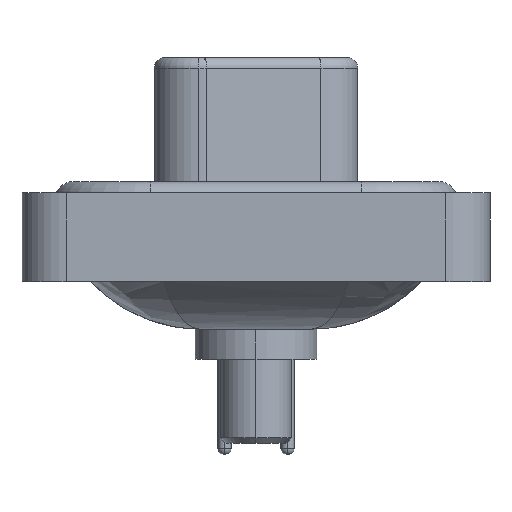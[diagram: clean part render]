
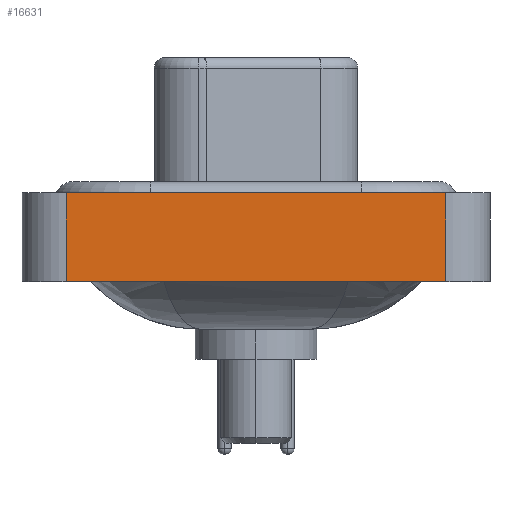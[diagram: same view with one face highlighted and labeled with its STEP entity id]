
A CAD part, left-side view. The second image highlights one B-rep face of the part: STEP entity #16631.
In plain terms, the highlighted planar face has unit normal (-1, 0, 0).
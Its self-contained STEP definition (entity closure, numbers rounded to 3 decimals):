
#291 = DIRECTION ( 'NONE',  ( -1., 0., 0. ) ) ;
#383 = VERTEX_POINT ( 'NONE', #11152 ) ;
#412 = CARTESIAN_POINT ( 'NONE',  ( -7.35, -8.55, -3.6 ) ) ;
#646 = DIRECTION ( 'NONE',  ( 0., 0., 1. ) ) ;
#1917 = VECTOR ( 'NONE', #2023, 1000. ) ;
#2023 = DIRECTION ( 'NONE',  ( 0., -1., 0. ) ) ;
#2479 = ORIENTED_EDGE ( 'NONE', *, *, #7269, .F. ) ;
#2492 = EDGE_CURVE ( 'NONE', #11780, #22816, #21795, .T. ) ;
#2498 = DIRECTION ( 'NONE',  ( 0., -1., 0. ) ) ;
#2768 = DIRECTION ( 'NONE',  ( 0., 0., 1. ) ) ;
#3832 = PLANE ( 'NONE',  #14014 ) ;
#6629 = VERTEX_POINT ( 'NONE', #16691 ) ;
#7155 = EDGE_LOOP ( 'NONE', ( #18305, #13038, #2479, #12317 ) ) ;
#7269 = EDGE_CURVE ( 'NONE', #11780, #6629, #9606, .T. ) ;
#7923 = EDGE_CURVE ( 'NONE', #6629, #383, #16283, .T. ) ;
#9606 = LINE ( 'NONE', #20671, #15294 ) ;
#10964 = CARTESIAN_POINT ( 'NONE',  ( -7.35, -8.55, -3.6 ) ) ;
#11152 = CARTESIAN_POINT ( 'NONE',  ( -7.35, -8.55, 0.4 ) ) ;
#11780 = VERTEX_POINT ( 'NONE', #14091 ) ;
#12317 = ORIENTED_EDGE ( 'NONE', *, *, #2492, .T. ) ;
#13038 = ORIENTED_EDGE ( 'NONE', *, *, #7923, .F. ) ;
#13344 = EDGE_CURVE ( 'NONE', #22816, #383, #16536, .T. ) ;
#14014 = AXIS2_PLACEMENT_3D ( 'NONE', #16430, #291, #2768 ) ;
#14091 = CARTESIAN_POINT ( 'NONE',  ( -7.35, 8.55, -3.6 ) ) ;
#14959 = CARTESIAN_POINT ( 'NONE',  ( -7.35, -8.55, 0.4 ) ) ;
#15044 = VECTOR ( 'NONE', #22304, 1000. ) ;
#15294 = VECTOR ( 'NONE', #646, 1000. ) ;
#15697 = VECTOR ( 'NONE', #2498, 1000. ) ;
#16283 = LINE ( 'NONE', #14959, #15697 ) ;
#16430 = CARTESIAN_POINT ( 'NONE',  ( -7.35, -8.55, -3.6 ) ) ;
#16536 = LINE ( 'NONE', #412, #15044 ) ;
#16631 = ADVANCED_FACE ( 'NONE', ( #21722 ), #3832, .T. ) ;
#16691 = CARTESIAN_POINT ( 'NONE',  ( -7.35, 8.55, 0.4 ) ) ;
#18305 = ORIENTED_EDGE ( 'NONE', *, *, #13344, .T. ) ;
#20671 = CARTESIAN_POINT ( 'NONE',  ( -7.35, 8.55, -3.6 ) ) ;
#21722 = FACE_OUTER_BOUND ( 'NONE', #7155, .T. ) ;
#21795 = LINE ( 'NONE', #10964, #1917 ) ;
#22238 = CARTESIAN_POINT ( 'NONE',  ( -7.35, -8.55, -3.6 ) ) ;
#22304 = DIRECTION ( 'NONE',  ( 0., 0., 1. ) ) ;
#22816 = VERTEX_POINT ( 'NONE', #22238 ) ;
